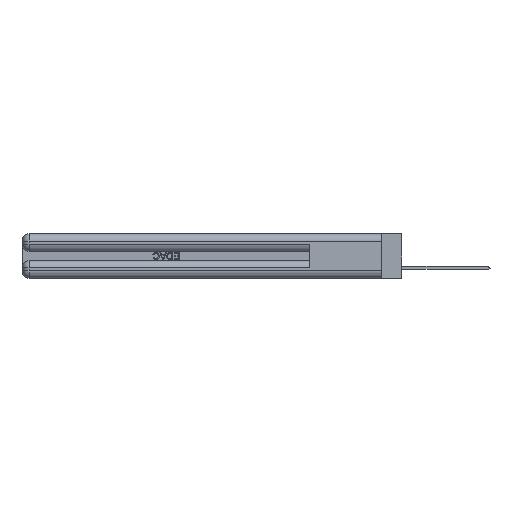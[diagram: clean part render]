
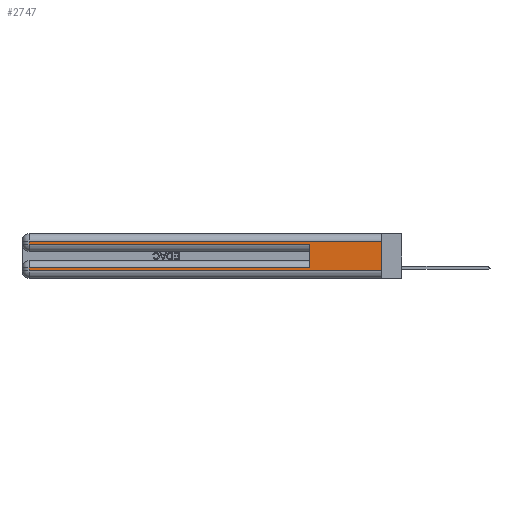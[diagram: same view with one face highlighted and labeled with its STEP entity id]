
A CAD part, left-side view. The second image highlights one B-rep face of the part: STEP entity #2747.
In plain terms, the highlighted planar face has unit normal (-1, 0, 0).
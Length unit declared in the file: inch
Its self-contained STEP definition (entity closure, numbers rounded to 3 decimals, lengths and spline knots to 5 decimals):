
#110 = ORIENTED_EDGE ( 'NONE', *, *, #50252, .T. ) ;
#959 = VECTOR ( 'NONE', #26923, 39.37008 ) ;
#1038 = ORIENTED_EDGE ( 'NONE', *, *, #37027, .F. ) ;
#2127 = CARTESIAN_POINT ( 'NONE',  ( 0., 0., 0.31 ) ) ;
#2727 = CARTESIAN_POINT ( 'NONE',  ( 0., 0., 0.285 ) ) ;
#2736 = ORIENTED_EDGE ( 'NONE', *, *, #33195, .T. ) ;
#2747 = ADVANCED_FACE ( 'NONE', ( #41857 ), #6731, .F. ) ;
#3651 = ORIENTED_EDGE ( 'NONE', *, *, #32011, .T. ) ;
#3724 = ORIENTED_EDGE ( 'NONE', *, *, #14117, .T. ) ;
#3993 = VERTEX_POINT ( 'NONE', #20534 ) ;
#4084 = DIRECTION ( 'NONE',  ( 0., -1., 0. ) ) ;
#4088 = VECTOR ( 'NONE', #18327, 39.37008 ) ;
#4339 = VERTEX_POINT ( 'NONE', #20304 ) ;
#4528 = EDGE_CURVE ( 'NONE', #23934, #29600, #25641, .T. ) ;
#6677 = LINE ( 'NONE', #39392, #9115 ) ;
#6731 = PLANE ( 'NONE',  #31177 ) ;
#8866 = CARTESIAN_POINT ( 'NONE',  ( 0., 0.6, 0.085 ) ) ;
#9115 = VECTOR ( 'NONE', #4084, 39.37008 ) ;
#10440 = VECTOR ( 'NONE', #24723, 39.37008 ) ;
#10522 = ORIENTED_EDGE ( 'NONE', *, *, #20775, .F. ) ;
#11078 = DIRECTION ( 'NONE',  ( 0., 0., -1. ) ) ;
#14117 = EDGE_CURVE ( 'NONE', #49199, #37911, #28808, .T. ) ;
#14565 = LINE ( 'NONE', #27380, #45955 ) ;
#15279 = EDGE_LOOP ( 'NONE', ( #10522, #27879, #3651, #41759, #1038, #3724, #2736, #110 ) ) ;
#18071 = CARTESIAN_POINT ( 'NONE',  ( 0., 2.94, 0.085 ) ) ;
#18327 = DIRECTION ( 'NONE',  ( 0., 0., -1. ) ) ;
#18851 = VERTEX_POINT ( 'NONE', #47946 ) ;
#19303 = DIRECTION ( 'NONE',  ( 0., 0., -1. ) ) ;
#20304 = CARTESIAN_POINT ( 'NONE',  ( 0., 2.94, 0.31 ) ) ;
#20534 = CARTESIAN_POINT ( 'NONE',  ( 0., 0., 0.06 ) ) ;
#20775 = EDGE_CURVE ( 'NONE', #18851, #3993, #48951, .T. ) ;
#22450 = LINE ( 'NONE', #46103, #23662 ) ;
#23014 = VECTOR ( 'NONE', #19303, 39.37008 ) ;
#23098 = DIRECTION ( 'NONE',  ( 1., 0., 0. ) ) ;
#23662 = VECTOR ( 'NONE', #42831, 39.37008 ) ;
#23934 = VERTEX_POINT ( 'NONE', #40917 ) ;
#24723 = DIRECTION ( 'NONE',  ( 0., 1., 0. ) ) ;
#25641 = LINE ( 'NONE', #2727, #959 ) ;
#26923 = DIRECTION ( 'NONE',  ( 0., -1., 0. ) ) ;
#27380 = CARTESIAN_POINT ( 'NONE',  ( 0., 0.6, 0.145 ) ) ;
#27879 = ORIENTED_EDGE ( 'NONE', *, *, #47879, .T. ) ;
#28808 = LINE ( 'NONE', #51127, #48552 ) ;
#29600 = VERTEX_POINT ( 'NONE', #46185 ) ;
#31177 = AXIS2_PLACEMENT_3D ( 'NONE', #34317, #23098, #11078 ) ;
#31339 = LINE ( 'NONE', #2127, #10440 ) ;
#32011 = EDGE_CURVE ( 'NONE', #4339, #23934, #46624, .T. ) ;
#32301 = DIRECTION ( 'NONE',  ( 0., 1., 0. ) ) ;
#33195 = EDGE_CURVE ( 'NONE', #37911, #47037, #22450, .T. ) ;
#34317 = CARTESIAN_POINT ( 'NONE',  ( 0., 0., 0.37 ) ) ;
#35547 = DIRECTION ( 'NONE',  ( 0., 0., 1. ) ) ;
#37027 = EDGE_CURVE ( 'NONE', #49199, #29600, #14565, .T. ) ;
#37911 = VERTEX_POINT ( 'NONE', #18071 ) ;
#38609 = CARTESIAN_POINT ( 'NONE',  ( 0., 0., 0.37 ) ) ;
#39392 = CARTESIAN_POINT ( 'NONE',  ( 0., 0., 0.06 ) ) ;
#40917 = CARTESIAN_POINT ( 'NONE',  ( 0., 2.94, 0.285 ) ) ;
#41759 = ORIENTED_EDGE ( 'NONE', *, *, #4528, .T. ) ;
#41857 = FACE_OUTER_BOUND ( 'NONE', #15279, .T. ) ;
#42831 = DIRECTION ( 'NONE',  ( 0., 0., -1. ) ) ;
#45955 = VECTOR ( 'NONE', #35547, 39.37008 ) ;
#46103 = CARTESIAN_POINT ( 'NONE',  ( 0., 2.94, 0.37 ) ) ;
#46185 = CARTESIAN_POINT ( 'NONE',  ( 0., 0.6, 0.285 ) ) ;
#46624 = LINE ( 'NONE', #48323, #4088 ) ;
#47037 = VERTEX_POINT ( 'NONE', #47964 ) ;
#47879 = EDGE_CURVE ( 'NONE', #18851, #4339, #31339, .T. ) ;
#47946 = CARTESIAN_POINT ( 'NONE',  ( 0., 0., 0.31 ) ) ;
#47964 = CARTESIAN_POINT ( 'NONE',  ( 0., 2.94, 0.06 ) ) ;
#48323 = CARTESIAN_POINT ( 'NONE',  ( 0., 2.94, 0.37 ) ) ;
#48552 = VECTOR ( 'NONE', #32301, 39.37008 ) ;
#48951 = LINE ( 'NONE', #38609, #23014 ) ;
#49199 = VERTEX_POINT ( 'NONE', #8866 ) ;
#50252 = EDGE_CURVE ( 'NONE', #47037, #3993, #6677, .T. ) ;
#51127 = CARTESIAN_POINT ( 'NONE',  ( 0., 0., 0.085 ) ) ;
